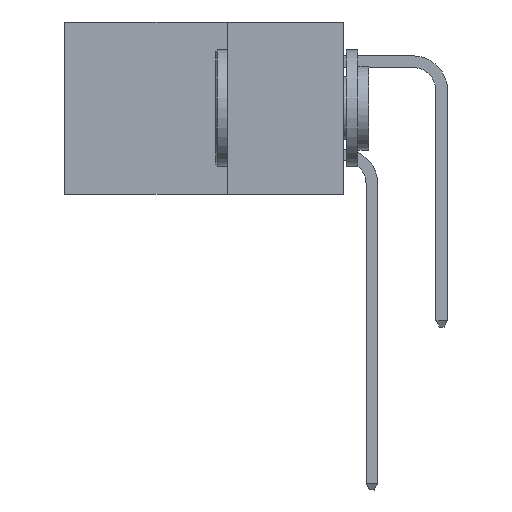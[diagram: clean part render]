
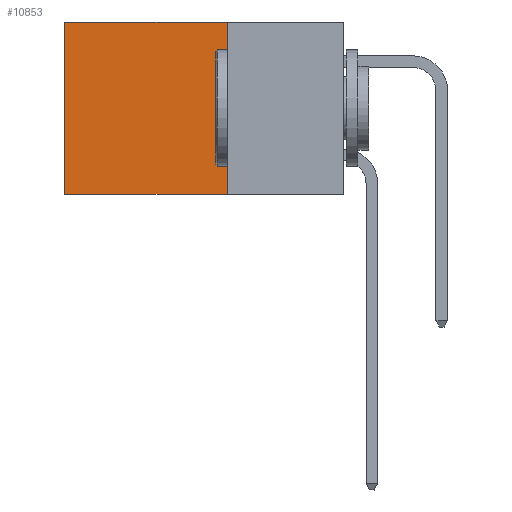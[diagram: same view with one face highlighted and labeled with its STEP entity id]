
A CAD part, left-side view. The second image highlights one B-rep face of the part: STEP entity #10853.
In plain terms, the highlighted planar face has unit normal (-1, 0, 0).
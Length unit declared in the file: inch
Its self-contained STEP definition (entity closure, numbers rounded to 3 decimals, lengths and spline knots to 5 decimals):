
#407 = CARTESIAN_POINT ( 'NONE',  ( 0.2615, 0.25, -0.37 ) ) ;
#739 = CARTESIAN_POINT ( 'NONE',  ( 0.2615, 0.25, -0.37 ) ) ;
#1254 = ORIENTED_EDGE ( 'NONE', *, *, #16548, .F. ) ;
#1769 = EDGE_CURVE ( 'NONE', #3979, #8343, #12390, .T. ) ;
#1831 = VECTOR ( 'NONE', #18042, 39.37008 ) ;
#2249 = EDGE_CURVE ( 'NONE', #9487, #3979, #12921, .T. ) ;
#2317 = CARTESIAN_POINT ( 'NONE',  ( 0.2615, 0.6, -0.37 ) ) ;
#2428 = VERTEX_POINT ( 'NONE', #13565 ) ;
#2606 = EDGE_LOOP ( 'NONE', ( #7193, #1254, #8746, #9543 ) ) ;
#2649 = AXIS2_PLACEMENT_3D ( 'NONE', #11364, #9781, #5350 ) ;
#3665 = VECTOR ( 'NONE', #12847, 39.37008 ) ;
#3979 = VERTEX_POINT ( 'NONE', #7438 ) ;
#4102 = FACE_OUTER_BOUND ( 'NONE', #2606, .T. ) ;
#4225 = CARTESIAN_POINT ( 'NONE',  ( 0.2615, 0.25, 0. ) ) ;
#5350 = DIRECTION ( 'NONE',  ( 0., 0., -1. ) ) ;
#6256 = DIRECTION ( 'NONE',  ( 0., 0., -1. ) ) ;
#6855 = EDGE_CURVE ( 'NONE', #9487, #2428, #14918, .T. ) ;
#7193 = ORIENTED_EDGE ( 'NONE', *, *, #1769, .T. ) ;
#7438 = CARTESIAN_POINT ( 'NONE',  ( 0.2615, 0.6, 0. ) ) ;
#8343 = VERTEX_POINT ( 'NONE', #16559 ) ;
#8746 = ORIENTED_EDGE ( 'NONE', *, *, #6855, .F. ) ;
#9487 = VERTEX_POINT ( 'NONE', #17929 ) ;
#9543 = ORIENTED_EDGE ( 'NONE', *, *, #2249, .T. ) ;
#9690 = PLANE ( 'NONE',  #2649 ) ;
#9781 = DIRECTION ( 'NONE',  ( 1., 0., 0. ) ) ;
#9908 = VECTOR ( 'NONE', #6256, 39.37008 ) ;
#10853 = ADVANCED_FACE ( 'NONE', ( #4102 ), #9690, .F. ) ;
#10878 = DIRECTION ( 'NONE',  ( 0., 1., 0. ) ) ;
#11364 = CARTESIAN_POINT ( 'NONE',  ( 0.2615, 0.25, -0.37 ) ) ;
#12390 = LINE ( 'NONE', #2317, #1831 ) ;
#12847 = DIRECTION ( 'NONE',  ( 0., 1., 0. ) ) ;
#12921 = LINE ( 'NONE', #4225, #3665 ) ;
#13565 = CARTESIAN_POINT ( 'NONE',  ( 0.2615, 0.25, -0.37 ) ) ;
#14918 = LINE ( 'NONE', #407, #9908 ) ;
#16548 = EDGE_CURVE ( 'NONE', #2428, #8343, #18172, .T. ) ;
#16559 = CARTESIAN_POINT ( 'NONE',  ( 0.2615, 0.6, -0.37 ) ) ;
#17004 = VECTOR ( 'NONE', #10878, 39.37008 ) ;
#17929 = CARTESIAN_POINT ( 'NONE',  ( 0.2615, 0.25, 0. ) ) ;
#18042 = DIRECTION ( 'NONE',  ( 0., 0., -1. ) ) ;
#18172 = LINE ( 'NONE', #739, #17004 ) ;
